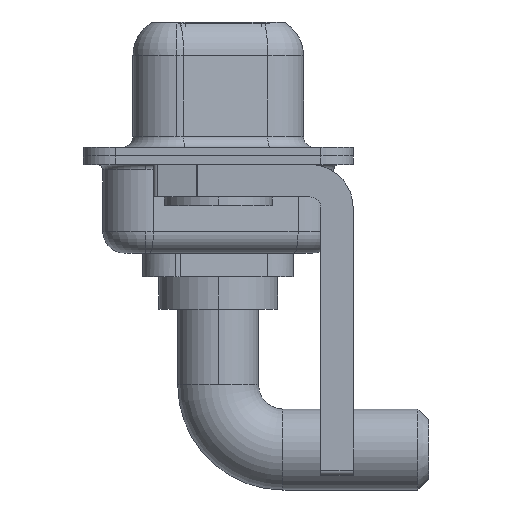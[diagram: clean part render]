
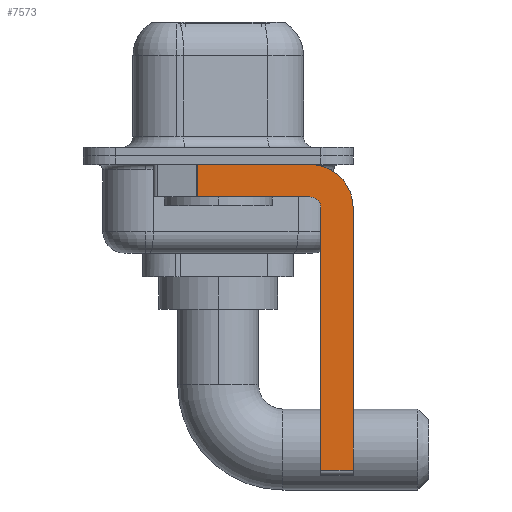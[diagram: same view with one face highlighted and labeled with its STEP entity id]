
A CAD part, left-side view. The second image highlights one B-rep face of the part: STEP entity #7573.
In plain terms, the highlighted planar face has unit normal (-1, 0, 0).
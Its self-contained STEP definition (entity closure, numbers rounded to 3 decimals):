
#53 = VECTOR ( 'NONE', #12378, 1000. ) ;
#61 = LINE ( 'NONE', #5039, #12538 ) ;
#311 = AXIS2_PLACEMENT_3D ( 'NONE', #1037, #10846, #7717 ) ;
#393 = VECTOR ( 'NONE', #3048, 1000. ) ;
#543 = DIRECTION ( 'NONE',  ( 1., 0., 0. ) ) ;
#755 = CARTESIAN_POINT ( 'NONE',  ( -2.9, -4.25, -2.4 ) ) ;
#900 = CARTESIAN_POINT ( 'NONE',  ( -2.9, -6.25, -2.4 ) ) ;
#1007 = CARTESIAN_POINT ( 'NONE',  ( -2.9, -4.25, -14.55 ) ) ;
#1037 = CARTESIAN_POINT ( 'NONE',  ( -2.9, -4.25, -2.4 ) ) ;
#1262 = CIRCLE ( 'NONE', #9777, 2. ) ;
#1336 = CARTESIAN_POINT ( 'NONE',  ( -2.9, -4.75, -2.4 ) ) ;
#1956 = DIRECTION ( 'NONE',  ( 0., -1., 0. ) ) ;
#2175 = LINE ( 'NONE', #900, #53 ) ;
#2267 = VERTEX_POINT ( 'NONE', #9223 ) ;
#2305 = EDGE_CURVE ( 'NONE', #7358, #3023, #1262, .T. ) ;
#2464 = EDGE_CURVE ( 'NONE', #4306, #10894, #6410, .T. ) ;
#3023 = VERTEX_POINT ( 'NONE', #5495 ) ;
#3048 = DIRECTION ( 'NONE',  ( 0., 0., 1. ) ) ;
#3094 = ORIENTED_EDGE ( 'NONE', *, *, #2305, .F. ) ;
#3170 = CARTESIAN_POINT ( 'NONE',  ( -2.9, -4.75, -14.55 ) ) ;
#3172 = DIRECTION ( 'NONE',  ( 0., -1., 0. ) ) ;
#3191 = ORIENTED_EDGE ( 'NONE', *, *, #10368, .F. ) ;
#3330 = CARTESIAN_POINT ( 'NONE',  ( -2.9, 0.978, -1.9 ) ) ;
#3750 = ORIENTED_EDGE ( 'NONE', *, *, #8686, .F. ) ;
#3805 = DIRECTION ( 'NONE',  ( 1., 0., 0. ) ) ;
#4021 = CIRCLE ( 'NONE', #311, 0.5 ) ;
#4306 = VERTEX_POINT ( 'NONE', #3170 ) ;
#4490 = EDGE_LOOP ( 'NONE', ( #13416, #7515, #3191, #6333, #7240, #12284, #3750, #3094 ) ) ;
#4694 = DIRECTION ( 'NONE',  ( 0., 0., -1. ) ) ;
#5039 = CARTESIAN_POINT ( 'NONE',  ( -2.9, 3., -0.4 ) ) ;
#5045 = AXIS2_PLACEMENT_3D ( 'NONE', #755, #543, #4694 ) ;
#5495 = CARTESIAN_POINT ( 'NONE',  ( -2.9, -6.25, -2.4 ) ) ;
#5755 = VECTOR ( 'NONE', #3172, 1000. ) ;
#5976 = VERTEX_POINT ( 'NONE', #12142 ) ;
#6079 = DIRECTION ( 'NONE',  ( 0., 1., 0. ) ) ;
#6333 = ORIENTED_EDGE ( 'NONE', *, *, #10844, .F. ) ;
#6410 = LINE ( 'NONE', #11661, #393 ) ;
#6976 = FACE_OUTER_BOUND ( 'NONE', #4490, .T. ) ;
#7049 = LINE ( 'NONE', #11203, #7974 ) ;
#7240 = ORIENTED_EDGE ( 'NONE', *, *, #2464, .F. ) ;
#7358 = VERTEX_POINT ( 'NONE', #12705 ) ;
#7515 = ORIENTED_EDGE ( 'NONE', *, *, #8673, .T. ) ;
#7573 = ADVANCED_FACE ( 'NONE', ( #6976 ), #10112, .F. ) ;
#7717 = DIRECTION ( 'NONE',  ( 0., 0., 1. ) ) ;
#7974 = VECTOR ( 'NONE', #6079, 1000. ) ;
#8347 = CARTESIAN_POINT ( 'NONE',  ( -2.9, -6.25, -14.55 ) ) ;
#8673 = EDGE_CURVE ( 'NONE', #2267, #8895, #11343, .T. ) ;
#8686 = EDGE_CURVE ( 'NONE', #3023, #9243, #2175, .T. ) ;
#8895 = VERTEX_POINT ( 'NONE', #3330 ) ;
#9223 = CARTESIAN_POINT ( 'NONE',  ( -2.9, 0.978, -0.4 ) ) ;
#9243 = VERTEX_POINT ( 'NONE', #8347 ) ;
#9436 = CARTESIAN_POINT ( 'NONE',  ( -2.9, 0.978, -1.9 ) ) ;
#9622 = EDGE_CURVE ( 'NONE', #4306, #9243, #10363, .T. ) ;
#9777 = AXIS2_PLACEMENT_3D ( 'NONE', #11198, #3805, #12229 ) ;
#10099 = VECTOR ( 'NONE', #11412, 1000. ) ;
#10112 = PLANE ( 'NONE',  #5045 ) ;
#10363 = LINE ( 'NONE', #1007, #5755 ) ;
#10368 = EDGE_CURVE ( 'NONE', #5976, #8895, #7049, .T. ) ;
#10485 = EDGE_CURVE ( 'NONE', #2267, #7358, #61, .T. ) ;
#10844 = EDGE_CURVE ( 'NONE', #10894, #5976, #4021, .T. ) ;
#10846 = DIRECTION ( 'NONE',  ( -1., 0., 0. ) ) ;
#10894 = VERTEX_POINT ( 'NONE', #1336 ) ;
#11198 = CARTESIAN_POINT ( 'NONE',  ( -2.9, -4.25, -2.4 ) ) ;
#11203 = CARTESIAN_POINT ( 'NONE',  ( -2.9, -4.25, -1.9 ) ) ;
#11343 = LINE ( 'NONE', #9436, #10099 ) ;
#11412 = DIRECTION ( 'NONE',  ( 0., 0., -1. ) ) ;
#11661 = CARTESIAN_POINT ( 'NONE',  ( -2.9, -4.75, -14.8 ) ) ;
#12142 = CARTESIAN_POINT ( 'NONE',  ( -2.9, -4.25, -1.9 ) ) ;
#12229 = DIRECTION ( 'NONE',  ( 0., 0., -1. ) ) ;
#12284 = ORIENTED_EDGE ( 'NONE', *, *, #9622, .T. ) ;
#12378 = DIRECTION ( 'NONE',  ( 0., 0., -1. ) ) ;
#12538 = VECTOR ( 'NONE', #1956, 1000. ) ;
#12705 = CARTESIAN_POINT ( 'NONE',  ( -2.9, -4.25, -0.4 ) ) ;
#13416 = ORIENTED_EDGE ( 'NONE', *, *, #10485, .F. ) ;
